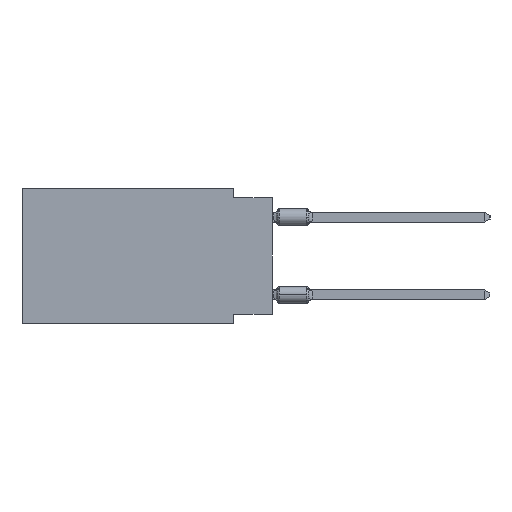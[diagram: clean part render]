
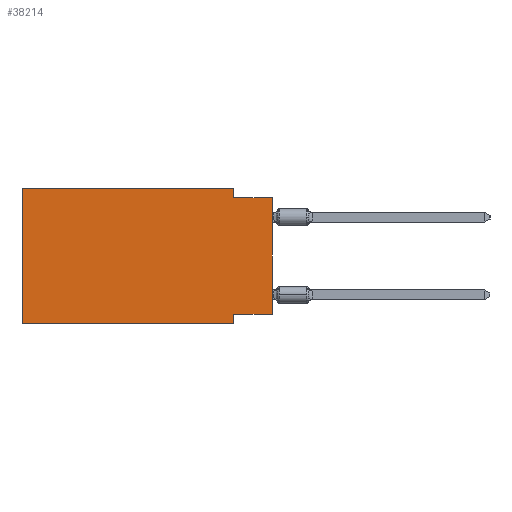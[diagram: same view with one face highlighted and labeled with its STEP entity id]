
A CAD part, left-side view. The second image highlights one B-rep face of the part: STEP entity #38214.
In plain terms, the highlighted planar face has unit normal (-1, 0, 0).
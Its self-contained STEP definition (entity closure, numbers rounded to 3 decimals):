
#3833 = DIRECTION ( 'NONE',  ( 0., 0., 1. ) ) ;
#6631 = CARTESIAN_POINT ( 'NONE',  ( 0., 0., -0.635 ) ) ;
#7088 = CARTESIAN_POINT ( 'NONE',  ( 0., 2.54, -8.255 ) ) ;
#7188 = CARTESIAN_POINT ( 'NONE',  ( 0., 2.54, 0. ) ) ;
#7863 = CARTESIAN_POINT ( 'NONE',  ( 0., 16.383, 0. ) ) ;
#8619 = EDGE_LOOP ( 'NONE', ( #22184, #23276, #39457, #12746, #11526, #21503, #12674, #42931 ) ) ;
#9329 = LINE ( 'NONE', #49124, #15989 ) ;
#10408 = CARTESIAN_POINT ( 'NONE',  ( 0., 0., -0.635 ) ) ;
#10743 = VECTOR ( 'NONE', #20293, 1000. ) ;
#11526 = ORIENTED_EDGE ( 'NONE', *, *, #55923, .F. ) ;
#12079 = LINE ( 'NONE', #59313, #17737 ) ;
#12674 = ORIENTED_EDGE ( 'NONE', *, *, #22620, .F. ) ;
#12746 = ORIENTED_EDGE ( 'NONE', *, *, #13497, .F. ) ;
#12866 = VECTOR ( 'NONE', #33032, 1000. ) ;
#13100 = PLANE ( 'NONE',  #48049 ) ;
#13497 = EDGE_CURVE ( 'NONE', #49431, #19093, #9329, .T. ) ;
#14219 = LINE ( 'NONE', #56486, #12866 ) ;
#15989 = VECTOR ( 'NONE', #30288, 1000. ) ;
#17163 = LINE ( 'NONE', #54807, #18445 ) ;
#17737 = VECTOR ( 'NONE', #40469, 1000. ) ;
#18445 = VECTOR ( 'NONE', #35971, 1000. ) ;
#18547 = EDGE_CURVE ( 'NONE', #34171, #37109, #17163, .T. ) ;
#19093 = VERTEX_POINT ( 'NONE', #7188 ) ;
#20293 = DIRECTION ( 'NONE',  ( 0., -1., 0. ) ) ;
#21503 = ORIENTED_EDGE ( 'NONE', *, *, #26388, .T. ) ;
#22077 = DIRECTION ( 'NONE',  ( 0., 0., -1. ) ) ;
#22184 = ORIENTED_EDGE ( 'NONE', *, *, #40347, .T. ) ;
#22380 = DIRECTION ( 'NONE',  ( 1., 0., 0. ) ) ;
#22620 = EDGE_CURVE ( 'NONE', #37109, #25042, #12079, .T. ) ;
#23276 = ORIENTED_EDGE ( 'NONE', *, *, #25037, .F. ) ;
#23702 = LINE ( 'NONE', #10408, #10743 ) ;
#24684 = CARTESIAN_POINT ( 'NONE',  ( 0., 16.383, -8.89 ) ) ;
#25037 = EDGE_CURVE ( 'NONE', #27441, #47814, #23702, .T. ) ;
#25042 = VERTEX_POINT ( 'NONE', #52408 ) ;
#25929 = DIRECTION ( 'NONE',  ( 0., 0., 1. ) ) ;
#26388 = EDGE_CURVE ( 'NONE', #26537, #25042, #14219, .T. ) ;
#26537 = VERTEX_POINT ( 'NONE', #24684 ) ;
#27149 = CARTESIAN_POINT ( 'NONE',  ( 0., 0., 0. ) ) ;
#27441 = VERTEX_POINT ( 'NONE', #55306 ) ;
#30288 = DIRECTION ( 'NONE',  ( 0., -1., 0. ) ) ;
#33032 = DIRECTION ( 'NONE',  ( 0., -1., 0. ) ) ;
#34171 = VERTEX_POINT ( 'NONE', #57543 ) ;
#35847 = VECTOR ( 'NONE', #48576, 1000. ) ;
#35941 = CARTESIAN_POINT ( 'NONE',  ( 0., 16.383, 0. ) ) ;
#35971 = DIRECTION ( 'NONE',  ( 0., 1., 0. ) ) ;
#37109 = VERTEX_POINT ( 'NONE', #7088 ) ;
#38214 = ADVANCED_FACE ( 'NONE', ( #39965 ), #13100, .F. ) ;
#39457 = ORIENTED_EDGE ( 'NONE', *, *, #51823, .F. ) ;
#39965 = FACE_OUTER_BOUND ( 'NONE', #8619, .T. ) ;
#40347 = EDGE_CURVE ( 'NONE', #34171, #47814, #45380, .T. ) ;
#40469 = DIRECTION ( 'NONE',  ( 0., 0., -1. ) ) ;
#42931 = ORIENTED_EDGE ( 'NONE', *, *, #18547, .F. ) ;
#45380 = LINE ( 'NONE', #27149, #46303 ) ;
#45521 = LINE ( 'NONE', #35941, #53723 ) ;
#46303 = VECTOR ( 'NONE', #25929, 1000. ) ;
#47814 = VERTEX_POINT ( 'NONE', #6631 ) ;
#48049 = AXIS2_PLACEMENT_3D ( 'NONE', #7863, #22380, #22077 ) ;
#48576 = DIRECTION ( 'NONE',  ( 0., 0., -1. ) ) ;
#49124 = CARTESIAN_POINT ( 'NONE',  ( 0., 16.383, 0. ) ) ;
#49431 = VERTEX_POINT ( 'NONE', #51456 ) ;
#51456 = CARTESIAN_POINT ( 'NONE',  ( 0., 16.383, 0. ) ) ;
#51823 = EDGE_CURVE ( 'NONE', #19093, #27441, #52910, .T. ) ;
#52408 = CARTESIAN_POINT ( 'NONE',  ( 0., 2.54, -8.89 ) ) ;
#52910 = LINE ( 'NONE', #57839, #35847 ) ;
#53723 = VECTOR ( 'NONE', #3833, 1000. ) ;
#54807 = CARTESIAN_POINT ( 'NONE',  ( 0., 0., -8.255 ) ) ;
#55306 = CARTESIAN_POINT ( 'NONE',  ( 0., 2.54, -0.635 ) ) ;
#55923 = EDGE_CURVE ( 'NONE', #26537, #49431, #45521, .T. ) ;
#56486 = CARTESIAN_POINT ( 'NONE',  ( 0., 16.383, -8.89 ) ) ;
#57543 = CARTESIAN_POINT ( 'NONE',  ( 0., 0., -8.255 ) ) ;
#57839 = CARTESIAN_POINT ( 'NONE',  ( 0., 2.54, 0. ) ) ;
#59313 = CARTESIAN_POINT ( 'NONE',  ( 0., 2.54, -8.89 ) ) ;
